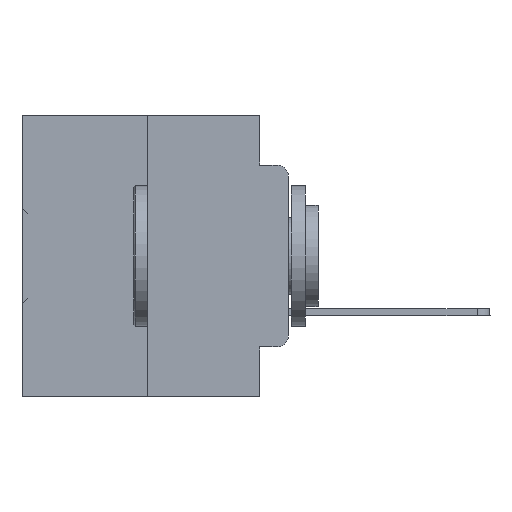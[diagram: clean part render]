
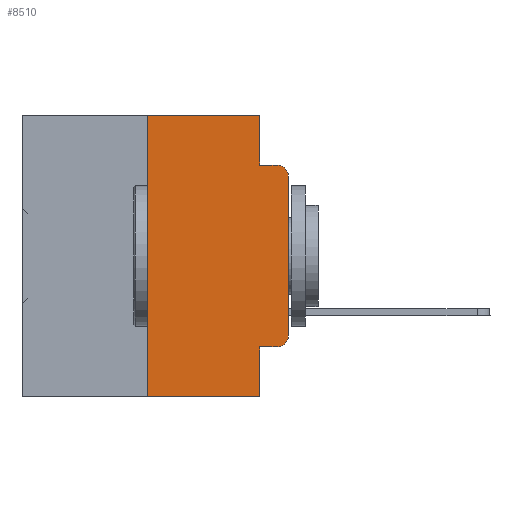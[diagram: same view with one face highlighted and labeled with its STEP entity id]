
A CAD part, left-side view. The second image highlights one B-rep face of the part: STEP entity #8510.
In plain terms, the highlighted planar face has unit normal (-1, 0, 0).
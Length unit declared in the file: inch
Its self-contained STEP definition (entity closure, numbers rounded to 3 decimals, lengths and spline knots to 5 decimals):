
#1645 = LINE ( 'NONE', #10381, #21803 ) ;
#2145 = EDGE_CURVE ( 'NONE', #25728, #35295, #13675, .T. ) ;
#2251 = CARTESIAN_POINT ( 'NONE',  ( 0., 0.25, 0. ) ) ;
#2498 = AXIS2_PLACEMENT_3D ( 'NONE', #15091, #26207, #9984 ) ;
#4359 = VECTOR ( 'NONE', #35719, 39.37008 ) ;
#4495 = AXIS2_PLACEMENT_3D ( 'NONE', #35840, #19064, #8291 ) ;
#4822 = VERTEX_POINT ( 'NONE', #16161 ) ;
#4839 = EDGE_CURVE ( 'NONE', #12612, #5779, #17291, .T. ) ;
#5093 = LINE ( 'NONE', #23815, #27399 ) ;
#5095 = CARTESIAN_POINT ( 'NONE',  ( 0., 0.051, 0. ) ) ;
#5779 = VERTEX_POINT ( 'NONE', #2251 ) ;
#6284 = EDGE_CURVE ( 'NONE', #4822, #15101, #23375, .T. ) ;
#6614 = ORIENTED_EDGE ( 'NONE', *, *, #23757, .F. ) ;
#6725 = DIRECTION ( 'NONE',  ( 0., 0., -1. ) ) ;
#7125 = CARTESIAN_POINT ( 'NONE',  ( 0., 0.02, -0.0885 ) ) ;
#7642 = VERTEX_POINT ( 'NONE', #8662 ) ;
#7896 = LINE ( 'NONE', #30171, #4359 ) ;
#7916 = DIRECTION ( 'NONE',  ( 0., 0., -1. ) ) ;
#8074 = CARTESIAN_POINT ( 'NONE',  ( 0., 0.051, -0.5 ) ) ;
#8109 = EDGE_CURVE ( 'NONE', #12612, #18750, #7896, .T. ) ;
#8161 = DIRECTION ( 'NONE',  ( 0., -1., 0. ) ) ;
#8291 = DIRECTION ( 'NONE',  ( 0., 0., -1. ) ) ;
#8510 = ADVANCED_FACE ( 'NONE', ( #15732 ), #12552, .F. ) ;
#8525 = LINE ( 'NONE', #5095, #21668 ) ;
#8633 = ORIENTED_EDGE ( 'NONE', *, *, #13792, .T. ) ;
#8662 = CARTESIAN_POINT ( 'NONE',  ( 0., 0.02, -0.4115 ) ) ;
#8685 = VECTOR ( 'NONE', #8161, 39.37008 ) ;
#9124 = EDGE_CURVE ( 'NONE', #13968, #7642, #1645, .T. ) ;
#9984 = DIRECTION ( 'NONE',  ( 0., 0., -1. ) ) ;
#10381 = CARTESIAN_POINT ( 'NONE',  ( 0., 0.051, -0.4115 ) ) ;
#10665 = CARTESIAN_POINT ( 'NONE',  ( 0., 0.051, 0. ) ) ;
#10947 = EDGE_CURVE ( 'NONE', #13968, #18750, #8525, .T. ) ;
#11132 = CARTESIAN_POINT ( 'NONE',  ( 0., 0.25, 0. ) ) ;
#11335 = CARTESIAN_POINT ( 'NONE',  ( 0., 0.02, -0.3915 ) ) ;
#12181 = EDGE_LOOP ( 'NONE', ( #14562, #24485, #14100, #6614, #31455, #20158, #23077, #25716, #35091, #8633 ) ) ;
#12552 = PLANE ( 'NONE',  #2498 ) ;
#12612 = VERTEX_POINT ( 'NONE', #28097 ) ;
#12663 = LINE ( 'NONE', #22317, #8685 ) ;
#13675 = LINE ( 'NONE', #35333, #25482 ) ;
#13792 = EDGE_CURVE ( 'NONE', #7642, #4822, #22754, .T. ) ;
#13968 = VERTEX_POINT ( 'NONE', #15822 ) ;
#14100 = ORIENTED_EDGE ( 'NONE', *, *, #2145, .F. ) ;
#14562 = ORIENTED_EDGE ( 'NONE', *, *, #6284, .T. ) ;
#15091 = CARTESIAN_POINT ( 'NONE',  ( 0., 0.473, 0. ) ) ;
#15101 = VERTEX_POINT ( 'NONE', #18024 ) ;
#15732 = FACE_OUTER_BOUND ( 'NONE', #12181, .T. ) ;
#15822 = CARTESIAN_POINT ( 'NONE',  ( 0., 0.051, -0.4115 ) ) ;
#15971 = VECTOR ( 'NONE', #29831, 39.37008 ) ;
#16161 = CARTESIAN_POINT ( 'NONE',  ( 0., 0., -0.3915 ) ) ;
#16960 = DIRECTION ( 'NONE',  ( 0., 0., 1. ) ) ;
#17291 = LINE ( 'NONE', #11132, #32220 ) ;
#18024 = CARTESIAN_POINT ( 'NONE',  ( 0., 0., -0.1085 ) ) ;
#18750 = VERTEX_POINT ( 'NONE', #8074 ) ;
#19057 = DIRECTION ( 'NONE',  ( 0., -1., 0. ) ) ;
#19064 = DIRECTION ( 'NONE',  ( -1., 0., 0. ) ) ;
#20158 = ORIENTED_EDGE ( 'NONE', *, *, #4839, .F. ) ;
#21123 = DIRECTION ( 'NONE',  ( 0., -1., 0. ) ) ;
#21668 = VECTOR ( 'NONE', #7916, 39.37008 ) ;
#21803 = VECTOR ( 'NONE', #19057, 39.37008 ) ;
#22317 = CARTESIAN_POINT ( 'NONE',  ( 0., 0.473, 0. ) ) ;
#22754 = CIRCLE ( 'NONE', #25540, 0.02 ) ;
#23077 = ORIENTED_EDGE ( 'NONE', *, *, #8109, .T. ) ;
#23375 = LINE ( 'NONE', #24708, #15971 ) ;
#23757 = EDGE_CURVE ( 'NONE', #35343, #25728, #5093, .T. ) ;
#23815 = CARTESIAN_POINT ( 'NONE',  ( 0., 0.051, 0. ) ) ;
#24485 = ORIENTED_EDGE ( 'NONE', *, *, #31530, .T. ) ;
#24708 = CARTESIAN_POINT ( 'NONE',  ( 0., 0., 0. ) ) ;
#25482 = VECTOR ( 'NONE', #21123, 39.37008 ) ;
#25540 = AXIS2_PLACEMENT_3D ( 'NONE', #11335, #30865, #36090 ) ;
#25716 = ORIENTED_EDGE ( 'NONE', *, *, #10947, .F. ) ;
#25728 = VERTEX_POINT ( 'NONE', #36113 ) ;
#26207 = DIRECTION ( 'NONE',  ( 1., 0., 0. ) ) ;
#27399 = VECTOR ( 'NONE', #6725, 39.37008 ) ;
#28097 = CARTESIAN_POINT ( 'NONE',  ( 0., 0.25, -0.5 ) ) ;
#28168 = EDGE_CURVE ( 'NONE', #5779, #35343, #12663, .T. ) ;
#29831 = DIRECTION ( 'NONE',  ( 0., 0., 1. ) ) ;
#30171 = CARTESIAN_POINT ( 'NONE',  ( 0., 0.473, -0.5 ) ) ;
#30865 = DIRECTION ( 'NONE',  ( -1., 0., 0. ) ) ;
#31455 = ORIENTED_EDGE ( 'NONE', *, *, #28168, .F. ) ;
#31530 = EDGE_CURVE ( 'NONE', #15101, #35295, #32610, .T. ) ;
#32220 = VECTOR ( 'NONE', #16960, 39.37008 ) ;
#32610 = CIRCLE ( 'NONE', #4495, 0.02 ) ;
#35091 = ORIENTED_EDGE ( 'NONE', *, *, #9124, .T. ) ;
#35295 = VERTEX_POINT ( 'NONE', #7125 ) ;
#35333 = CARTESIAN_POINT ( 'NONE',  ( 0., 0.051, -0.0885 ) ) ;
#35343 = VERTEX_POINT ( 'NONE', #10665 ) ;
#35719 = DIRECTION ( 'NONE',  ( 0., -1., 0. ) ) ;
#35840 = CARTESIAN_POINT ( 'NONE',  ( 0., 0.02, -0.1085 ) ) ;
#36090 = DIRECTION ( 'NONE',  ( 0., 0., -1. ) ) ;
#36113 = CARTESIAN_POINT ( 'NONE',  ( 0., 0.051, -0.0885 ) ) ;
